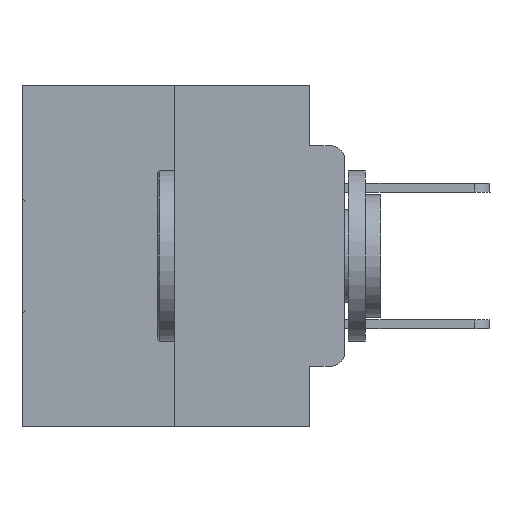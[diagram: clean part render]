
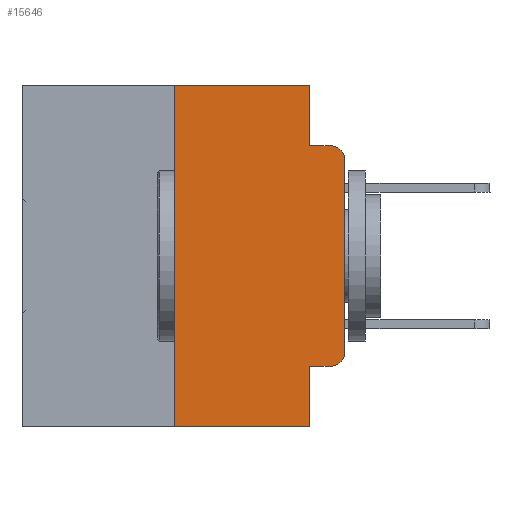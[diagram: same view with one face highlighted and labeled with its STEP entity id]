
A CAD part, left-side view. The second image highlights one B-rep face of the part: STEP entity #15646.
In plain terms, the highlighted planar face has unit normal (-1, 0, 0).
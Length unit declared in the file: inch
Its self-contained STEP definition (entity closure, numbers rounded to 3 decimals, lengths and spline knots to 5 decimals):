
#914 = CARTESIAN_POINT ( 'NONE',  ( 0., 0.02, -0.1085 ) ) ;
#1021 = DIRECTION ( 'NONE',  ( -1., 0., 0. ) ) ;
#1256 = ORIENTED_EDGE ( 'NONE', *, *, #32193, .T. ) ;
#1266 = EDGE_CURVE ( 'NONE', #17442, #20250, #14099, .T. ) ;
#1627 = AXIS2_PLACEMENT_3D ( 'NONE', #914, #1021, #23602 ) ;
#1732 = FACE_OUTER_BOUND ( 'NONE', #32113, .T. ) ;
#2148 = VECTOR ( 'NONE', #30286, 39.37008 ) ;
#2568 = LINE ( 'NONE', #27363, #31001 ) ;
#2852 = CARTESIAN_POINT ( 'NONE',  ( 0., 0.25, 0. ) ) ;
#2951 = CARTESIAN_POINT ( 'NONE',  ( 0., 0.051, 0. ) ) ;
#3074 = ORIENTED_EDGE ( 'NONE', *, *, #21514, .T. ) ;
#3645 = CARTESIAN_POINT ( 'NONE',  ( 0., 0.25, 0. ) ) ;
#3788 = CARTESIAN_POINT ( 'NONE',  ( 0., 0.25, -0.5 ) ) ;
#4390 = CARTESIAN_POINT ( 'NONE',  ( 0., 0.02, -0.3915 ) ) ;
#4802 = DIRECTION ( 'NONE',  ( 0., 0., 1. ) ) ;
#4990 = VECTOR ( 'NONE', #4802, 39.37008 ) ;
#5156 = VERTEX_POINT ( 'NONE', #20036 ) ;
#5226 = CARTESIAN_POINT ( 'NONE',  ( 0., 0., 0. ) ) ;
#5328 = DIRECTION ( 'NONE',  ( 1., 0., 0. ) ) ;
#5608 = DIRECTION ( 'NONE',  ( 0., 0., 1. ) ) ;
#6066 = VECTOR ( 'NONE', #27156, 39.37008 ) ;
#7134 = VERTEX_POINT ( 'NONE', #26760 ) ;
#7252 = EDGE_CURVE ( 'NONE', #5156, #10321, #27248, .T. ) ;
#8230 = CARTESIAN_POINT ( 'NONE',  ( 0., 0.051, 0. ) ) ;
#8233 = VERTEX_POINT ( 'NONE', #28407 ) ;
#9735 = VECTOR ( 'NONE', #30979, 39.37008 ) ;
#10118 = EDGE_CURVE ( 'NONE', #8233, #22386, #32096, .T. ) ;
#10321 = VERTEX_POINT ( 'NONE', #14010 ) ;
#10376 = CARTESIAN_POINT ( 'NONE',  ( 0., 0.473, 0. ) ) ;
#11044 = VECTOR ( 'NONE', #5608, 39.37008 ) ;
#11516 = CARTESIAN_POINT ( 'NONE',  ( 0., 0.051, -0.4115 ) ) ;
#13075 = LINE ( 'NONE', #31386, #15360 ) ;
#13274 = CARTESIAN_POINT ( 'NONE',  ( 0., 0.02, -0.0885 ) ) ;
#14010 = CARTESIAN_POINT ( 'NONE',  ( 0., 0.02, -0.4115 ) ) ;
#14099 = LINE ( 'NONE', #25120, #21106 ) ;
#14377 = LINE ( 'NONE', #5226, #4990 ) ;
#14691 = EDGE_CURVE ( 'NONE', #5156, #20547, #13075, .T. ) ;
#14776 = ORIENTED_EDGE ( 'NONE', *, *, #16281, .F. ) ;
#15360 = VECTOR ( 'NONE', #26701, 39.37008 ) ;
#15376 = DIRECTION ( 'NONE',  ( 0., -1., 0. ) ) ;
#15623 = EDGE_CURVE ( 'NONE', #20250, #7134, #20833, .T. ) ;
#15646 = ADVANCED_FACE ( 'NONE', ( #1732 ), #20301, .F. ) ;
#16281 = EDGE_CURVE ( 'NONE', #23775, #17442, #25457, .T. ) ;
#16932 = DIRECTION ( 'NONE',  ( -1., 0., 0. ) ) ;
#17047 = AXIS2_PLACEMENT_3D ( 'NONE', #4390, #16932, #29250 ) ;
#17442 = VERTEX_POINT ( 'NONE', #2852 ) ;
#19660 = ORIENTED_EDGE ( 'NONE', *, *, #10118, .T. ) ;
#20036 = CARTESIAN_POINT ( 'NONE',  ( 0., 0.051, -0.4115 ) ) ;
#20122 = DIRECTION ( 'NONE',  ( 0., -1., 0. ) ) ;
#20197 = DIRECTION ( 'NONE',  ( 0., 0., -1. ) ) ;
#20250 = VERTEX_POINT ( 'NONE', #8230 ) ;
#20301 = PLANE ( 'NONE',  #31990 ) ;
#20547 = VERTEX_POINT ( 'NONE', #26509 ) ;
#20833 = LINE ( 'NONE', #2951, #2148 ) ;
#21106 = VECTOR ( 'NONE', #20122, 39.37008 ) ;
#21305 = LINE ( 'NONE', #32060, #6066 ) ;
#21514 = EDGE_CURVE ( 'NONE', #23775, #20547, #21305, .T. ) ;
#21648 = EDGE_CURVE ( 'NONE', #7134, #22386, #2568, .T. ) ;
#22386 = VERTEX_POINT ( 'NONE', #13274 ) ;
#23602 = DIRECTION ( 'NONE',  ( 0., 0., -1. ) ) ;
#23775 = VERTEX_POINT ( 'NONE', #3788 ) ;
#24381 = ORIENTED_EDGE ( 'NONE', *, *, #14691, .F. ) ;
#25120 = CARTESIAN_POINT ( 'NONE',  ( 0., 0.473, 0. ) ) ;
#25457 = LINE ( 'NONE', #3645, #11044 ) ;
#25950 = ORIENTED_EDGE ( 'NONE', *, *, #15623, .F. ) ;
#26509 = CARTESIAN_POINT ( 'NONE',  ( 0., 0.051, -0.5 ) ) ;
#26701 = DIRECTION ( 'NONE',  ( 0., 0., -1. ) ) ;
#26760 = CARTESIAN_POINT ( 'NONE',  ( 0., 0.051, -0.0885 ) ) ;
#27113 = CARTESIAN_POINT ( 'NONE',  ( 0., 0., -0.3915 ) ) ;
#27156 = DIRECTION ( 'NONE',  ( 0., -1., 0. ) ) ;
#27248 = LINE ( 'NONE', #11516, #9735 ) ;
#27363 = CARTESIAN_POINT ( 'NONE',  ( 0., 0.051, -0.0885 ) ) ;
#27467 = ORIENTED_EDGE ( 'NONE', *, *, #1266, .F. ) ;
#28407 = CARTESIAN_POINT ( 'NONE',  ( 0., 0., -0.1085 ) ) ;
#28600 = EDGE_CURVE ( 'NONE', #29238, #8233, #14377, .T. ) ;
#29238 = VERTEX_POINT ( 'NONE', #27113 ) ;
#29250 = DIRECTION ( 'NONE',  ( 0., 0., -1. ) ) ;
#29846 = ORIENTED_EDGE ( 'NONE', *, *, #7252, .T. ) ;
#29969 = ORIENTED_EDGE ( 'NONE', *, *, #21648, .F. ) ;
#30286 = DIRECTION ( 'NONE',  ( 0., 0., -1. ) ) ;
#30509 = CIRCLE ( 'NONE', #17047, 0.02 ) ;
#30979 = DIRECTION ( 'NONE',  ( 0., -1., 0. ) ) ;
#31001 = VECTOR ( 'NONE', #15376, 39.37008 ) ;
#31386 = CARTESIAN_POINT ( 'NONE',  ( 0., 0.051, 0. ) ) ;
#31606 = ORIENTED_EDGE ( 'NONE', *, *, #28600, .T. ) ;
#31990 = AXIS2_PLACEMENT_3D ( 'NONE', #10376, #5328, #20197 ) ;
#32060 = CARTESIAN_POINT ( 'NONE',  ( 0., 0.473, -0.5 ) ) ;
#32096 = CIRCLE ( 'NONE', #1627, 0.02 ) ;
#32113 = EDGE_LOOP ( 'NONE', ( #31606, #19660, #29969, #25950, #27467, #14776, #3074, #24381, #29846, #1256 ) ) ;
#32193 = EDGE_CURVE ( 'NONE', #10321, #29238, #30509, .T. ) ;
